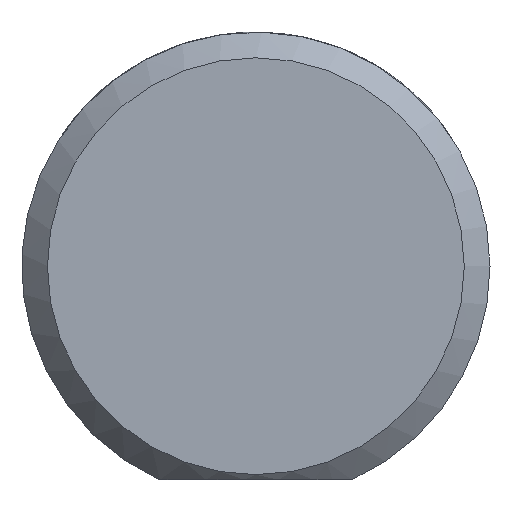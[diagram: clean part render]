
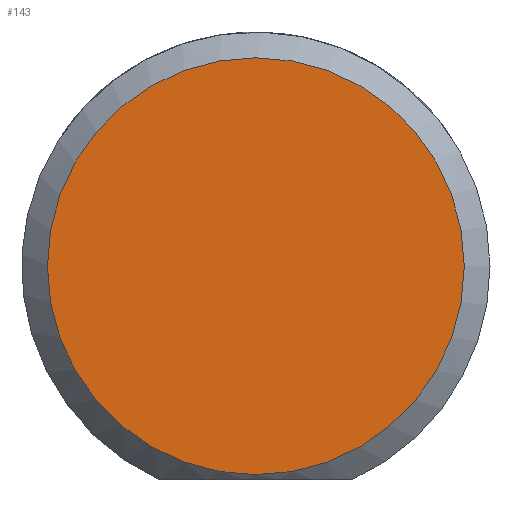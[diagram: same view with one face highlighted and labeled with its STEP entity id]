
A CAD part, front view. The second image highlights one B-rep face of the part: STEP entity #143.
In plain terms, the highlighted planar face has unit normal (0, -1, 0).
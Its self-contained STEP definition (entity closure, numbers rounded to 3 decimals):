
#30=CIRCLE('',#172,4.05);
#38=FACE_OUTER_BOUND('',#49,.T.);
#49=EDGE_LOOP('',(#123));
#77=VERTEX_POINT('',#295);
#92=EDGE_CURVE('',#77,#77,#30,.T.);
#123=ORIENTED_EDGE('',*,*,#92,.F.);
#136=PLANE('',#173);
#143=ADVANCED_FACE('',(#38),#136,.T.);
#172=AXIS2_PLACEMENT_3D('',#296,#206,#207);
#173=AXIS2_PLACEMENT_3D('',#298,#209,#210);
#206=DIRECTION('center_axis',(0.,1.,0.));
#207=DIRECTION('ref_axis',(-1.,0.,0.));
#209=DIRECTION('center_axis',(0.,-1.,0.));
#210=DIRECTION('ref_axis',(-1.,0.,0.));
#295=CARTESIAN_POINT('',(78.307,-7.823,4.15));
#296=CARTESIAN_POINT('Origin',(74.257,-7.823,4.15));
#298=CARTESIAN_POINT('Origin',(74.257,-7.823,4.15));
